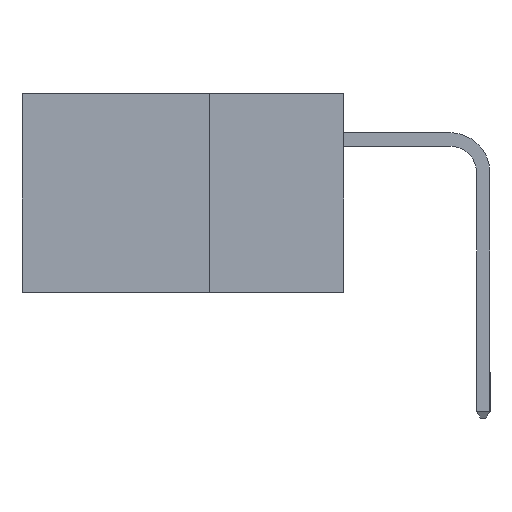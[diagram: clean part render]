
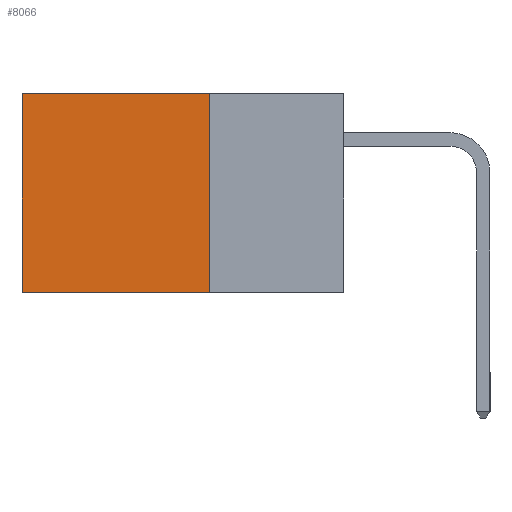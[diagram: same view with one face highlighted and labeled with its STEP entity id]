
A CAD part, left-side view. The second image highlights one B-rep face of the part: STEP entity #8066.
In plain terms, the highlighted planar face has unit normal (-1, 0, 0).
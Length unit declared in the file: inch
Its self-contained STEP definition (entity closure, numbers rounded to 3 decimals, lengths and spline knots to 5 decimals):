
#577 = FACE_OUTER_BOUND ( 'NONE', #7982, .T. ) ;
#593 = VERTEX_POINT ( 'NONE', #10513 ) ;
#784 = AXIS2_PLACEMENT_3D ( 'NONE', #10197, #12287, #9272 ) ;
#2008 = PLANE ( 'NONE',  #784 ) ;
#2099 = EDGE_CURVE ( 'NONE', #593, #10847, #5910, .T. ) ;
#2299 = LINE ( 'NONE', #5301, #7484 ) ;
#2343 = DIRECTION ( 'NONE',  ( 0., 0., -1. ) ) ;
#2702 = VECTOR ( 'NONE', #8011, 39.37008 ) ;
#3022 = CARTESIAN_POINT ( 'NONE',  ( 0.298, 0.6, 0. ) ) ;
#3309 = LINE ( 'NONE', #5747, #8493 ) ;
#4296 = CARTESIAN_POINT ( 'NONE',  ( 0.298, 0.25, 0. ) ) ;
#5301 = CARTESIAN_POINT ( 'NONE',  ( 0.298, 0.25, 0. ) ) ;
#5350 = VERTEX_POINT ( 'NONE', #10189 ) ;
#5747 = CARTESIAN_POINT ( 'NONE',  ( 0.298, 0.25, -0.37 ) ) ;
#5860 = VECTOR ( 'NONE', #11535, 39.37008 ) ;
#5910 = LINE ( 'NONE', #3022, #2702 ) ;
#7084 = ORIENTED_EDGE ( 'NONE', *, *, #11512, .F. ) ;
#7484 = VECTOR ( 'NONE', #2343, 39.37008 ) ;
#7799 = CARTESIAN_POINT ( 'NONE',  ( 0.298, 0.6, -0.37 ) ) ;
#7982 = EDGE_LOOP ( 'NONE', ( #11067, #7084, #10640, #8551 ) ) ;
#8011 = DIRECTION ( 'NONE',  ( 0., 0., -1. ) ) ;
#8066 = ADVANCED_FACE ( 'NONE', ( #577 ), #2008, .F. ) ;
#8162 = LINE ( 'NONE', #4296, #5860 ) ;
#8493 = VECTOR ( 'NONE', #11932, 39.37008 ) ;
#8551 = ORIENTED_EDGE ( 'NONE', *, *, #11238, .T. ) ;
#9272 = DIRECTION ( 'NONE',  ( 0., 0., -1. ) ) ;
#9413 = CARTESIAN_POINT ( 'NONE',  ( 0.298, 0.25, -0.37 ) ) ;
#9951 = VERTEX_POINT ( 'NONE', #9413 ) ;
#10189 = CARTESIAN_POINT ( 'NONE',  ( 0.298, 0.25, 0. ) ) ;
#10197 = CARTESIAN_POINT ( 'NONE',  ( 0.298, 0.25, 0. ) ) ;
#10513 = CARTESIAN_POINT ( 'NONE',  ( 0.298, 0.6, 0. ) ) ;
#10640 = ORIENTED_EDGE ( 'NONE', *, *, #13121, .F. ) ;
#10847 = VERTEX_POINT ( 'NONE', #7799 ) ;
#11067 = ORIENTED_EDGE ( 'NONE', *, *, #2099, .T. ) ;
#11238 = EDGE_CURVE ( 'NONE', #5350, #593, #8162, .T. ) ;
#11512 = EDGE_CURVE ( 'NONE', #9951, #10847, #3309, .T. ) ;
#11535 = DIRECTION ( 'NONE',  ( 0., 1., 0. ) ) ;
#11932 = DIRECTION ( 'NONE',  ( 0., 1., 0. ) ) ;
#12287 = DIRECTION ( 'NONE',  ( 1., 0., 0. ) ) ;
#13121 = EDGE_CURVE ( 'NONE', #5350, #9951, #2299, .T. ) ;
